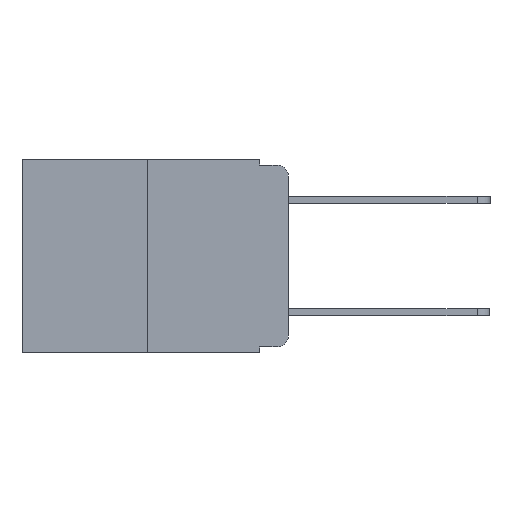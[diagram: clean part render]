
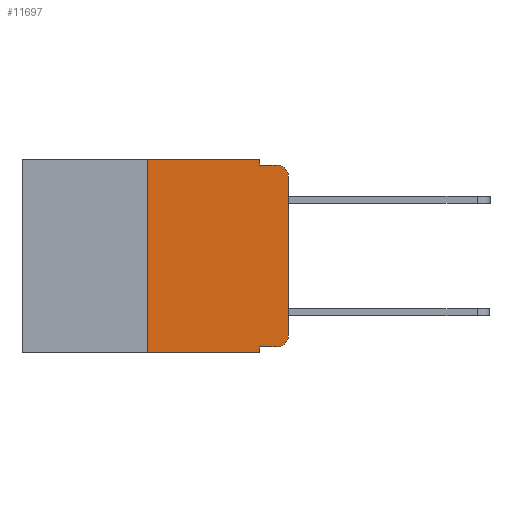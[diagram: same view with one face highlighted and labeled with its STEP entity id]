
A CAD part, left-side view. The second image highlights one B-rep face of the part: STEP entity #11697.
In plain terms, the highlighted planar face has unit normal (-1, 0, 0).
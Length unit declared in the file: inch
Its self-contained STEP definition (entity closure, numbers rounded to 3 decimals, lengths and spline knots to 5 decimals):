
#137 = CARTESIAN_POINT ( 'NONE',  ( 0., 0.473, -0.343 ) ) ;
#185 = DIRECTION ( 'NONE',  ( 0., 0., -1. ) ) ;
#206 = LINE ( 'NONE', #137, #13881 ) ;
#434 = DIRECTION ( 'NONE',  ( 0., -1., 0. ) ) ;
#602 = AXIS2_PLACEMENT_3D ( 'NONE', #12378, #7086, #19326 ) ;
#639 = DIRECTION ( 'NONE',  ( 0., 0., 1. ) ) ;
#973 = LINE ( 'NONE', #7373, #9947 ) ;
#1205 = VERTEX_POINT ( 'NONE', #8159 ) ;
#2012 = ORIENTED_EDGE ( 'NONE', *, *, #20556, .T. ) ;
#2899 = VERTEX_POINT ( 'NONE', #8703 ) ;
#3089 = VERTEX_POINT ( 'NONE', #12991 ) ;
#3859 = CARTESIAN_POINT ( 'NONE',  ( 0., 0.051, 0. ) ) ;
#4295 = VECTOR ( 'NONE', #22360, 39.37008 ) ;
#4531 = ORIENTED_EDGE ( 'NONE', *, *, #16497, .F. ) ;
#4762 = VECTOR ( 'NONE', #18342, 39.37008 ) ;
#4911 = EDGE_CURVE ( 'NONE', #16834, #7867, #18355, .T. ) ;
#5110 = ORIENTED_EDGE ( 'NONE', *, *, #13216, .T. ) ;
#5505 = VECTOR ( 'NONE', #18721, 39.37008 ) ;
#5928 = ORIENTED_EDGE ( 'NONE', *, *, #4911, .F. ) ;
#5935 = VERTEX_POINT ( 'NONE', #13872 ) ;
#7086 = DIRECTION ( 'NONE',  ( 1., 0., 0. ) ) ;
#7373 = CARTESIAN_POINT ( 'NONE',  ( 0., 0., 0. ) ) ;
#7867 = VERTEX_POINT ( 'NONE', #19276 ) ;
#8028 = CARTESIAN_POINT ( 'NONE',  ( 0., 0.02, -0.313 ) ) ;
#8159 = CARTESIAN_POINT ( 'NONE',  ( 0., 0., -0.313 ) ) ;
#8703 = CARTESIAN_POINT ( 'NONE',  ( 0., 0., -0.03 ) ) ;
#9113 = VECTOR ( 'NONE', #434, 39.37008 ) ;
#9176 = DIRECTION ( 'NONE',  ( 0., 0., 1. ) ) ;
#9227 = CARTESIAN_POINT ( 'NONE',  ( 0., 0.051, -0.343 ) ) ;
#9426 = CARTESIAN_POINT ( 'NONE',  ( 0., 0.25, 0. ) ) ;
#9532 = LINE ( 'NONE', #16645, #4762 ) ;
#9767 = CARTESIAN_POINT ( 'NONE',  ( 0., 0.25, -0.343 ) ) ;
#9798 = DIRECTION ( 'NONE',  ( 0., 0., -1. ) ) ;
#9947 = VECTOR ( 'NONE', #9176, 39.37008 ) ;
#10273 = LINE ( 'NONE', #21711, #18968 ) ;
#10498 = AXIS2_PLACEMENT_3D ( 'NONE', #21268, #10919, #185 ) ;
#10675 = CARTESIAN_POINT ( 'NONE',  ( 0., 0.051, -0.01 ) ) ;
#10919 = DIRECTION ( 'NONE',  ( -1., 0., 0. ) ) ;
#11013 = VERTEX_POINT ( 'NONE', #9426 ) ;
#11253 = ORIENTED_EDGE ( 'NONE', *, *, #20502, .F. ) ;
#11511 = ORIENTED_EDGE ( 'NONE', *, *, #12482, .T. ) ;
#11697 = ADVANCED_FACE ( 'NONE', ( #21871 ), #17617, .F. ) ;
#12378 = CARTESIAN_POINT ( 'NONE',  ( 0., 0.473, 0. ) ) ;
#12413 = AXIS2_PLACEMENT_3D ( 'NONE', #8028, #20209, #9798 ) ;
#12437 = DIRECTION ( 'NONE',  ( 0., -1., 0. ) ) ;
#12482 = EDGE_CURVE ( 'NONE', #1205, #2899, #973, .T. ) ;
#12683 = VERTEX_POINT ( 'NONE', #9767 ) ;
#12930 = CARTESIAN_POINT ( 'NONE',  ( 0., 0.051, -0.333 ) ) ;
#12991 = CARTESIAN_POINT ( 'NONE',  ( 0., 0.02, -0.01 ) ) ;
#13216 = EDGE_CURVE ( 'NONE', #15812, #5935, #22383, .T. ) ;
#13872 = CARTESIAN_POINT ( 'NONE',  ( 0., 0.02, -0.333 ) ) ;
#13881 = VECTOR ( 'NONE', #17863, 39.37008 ) ;
#14287 = ORIENTED_EDGE ( 'NONE', *, *, #19036, .F. ) ;
#14862 = CARTESIAN_POINT ( 'NONE',  ( 0., 0.051, -0.333 ) ) ;
#15363 = VECTOR ( 'NONE', #12437, 39.37008 ) ;
#15380 = ORIENTED_EDGE ( 'NONE', *, *, #18810, .F. ) ;
#15690 = VERTEX_POINT ( 'NONE', #9227 ) ;
#15812 = VERTEX_POINT ( 'NONE', #14862 ) ;
#15882 = CARTESIAN_POINT ( 'NONE',  ( 0., 0.051, 0. ) ) ;
#16497 = EDGE_CURVE ( 'NONE', #15812, #15690, #9532, .T. ) ;
#16645 = CARTESIAN_POINT ( 'NONE',  ( 0., 0.051, 0. ) ) ;
#16834 = VERTEX_POINT ( 'NONE', #15882 ) ;
#17017 = CARTESIAN_POINT ( 'NONE',  ( 0., 0.473, 0. ) ) ;
#17124 = CIRCLE ( 'NONE', #10498, 0.02 ) ;
#17534 = ORIENTED_EDGE ( 'NONE', *, *, #18008, .T. ) ;
#17617 = PLANE ( 'NONE',  #602 ) ;
#17863 = DIRECTION ( 'NONE',  ( 0., -1., 0. ) ) ;
#18008 = EDGE_CURVE ( 'NONE', #12683, #15690, #206, .T. ) ;
#18106 = EDGE_LOOP ( 'NONE', ( #11511, #22306, #14287, #5928, #15380, #11253, #17534, #4531, #5110, #2012 ) ) ;
#18342 = DIRECTION ( 'NONE',  ( 0., 0., -1. ) ) ;
#18355 = LINE ( 'NONE', #3859, #4295 ) ;
#18428 = CIRCLE ( 'NONE', #12413, 0.02 ) ;
#18721 = DIRECTION ( 'NONE',  ( 0., -1., 0. ) ) ;
#18810 = EDGE_CURVE ( 'NONE', #11013, #16834, #19493, .T. ) ;
#18968 = VECTOR ( 'NONE', #639, 39.37008 ) ;
#19036 = EDGE_CURVE ( 'NONE', #7867, #3089, #19215, .T. ) ;
#19215 = LINE ( 'NONE', #10675, #15363 ) ;
#19276 = CARTESIAN_POINT ( 'NONE',  ( 0., 0.051, -0.01 ) ) ;
#19326 = DIRECTION ( 'NONE',  ( 0., 0., -1. ) ) ;
#19493 = LINE ( 'NONE', #17017, #5505 ) ;
#20209 = DIRECTION ( 'NONE',  ( -1., 0., 0. ) ) ;
#20348 = EDGE_CURVE ( 'NONE', #2899, #3089, #17124, .T. ) ;
#20502 = EDGE_CURVE ( 'NONE', #12683, #11013, #10273, .T. ) ;
#20556 = EDGE_CURVE ( 'NONE', #5935, #1205, #18428, .T. ) ;
#21268 = CARTESIAN_POINT ( 'NONE',  ( 0., 0.02, -0.03 ) ) ;
#21711 = CARTESIAN_POINT ( 'NONE',  ( 0., 0.25, 0. ) ) ;
#21871 = FACE_OUTER_BOUND ( 'NONE', #18106, .T. ) ;
#22306 = ORIENTED_EDGE ( 'NONE', *, *, #20348, .T. ) ;
#22360 = DIRECTION ( 'NONE',  ( 0., 0., -1. ) ) ;
#22383 = LINE ( 'NONE', #12930, #9113 ) ;
